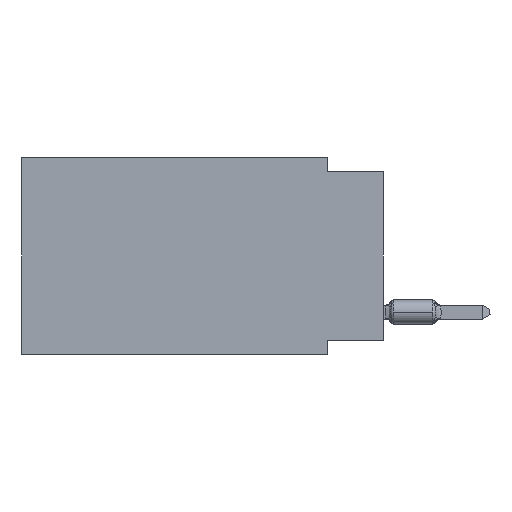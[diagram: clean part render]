
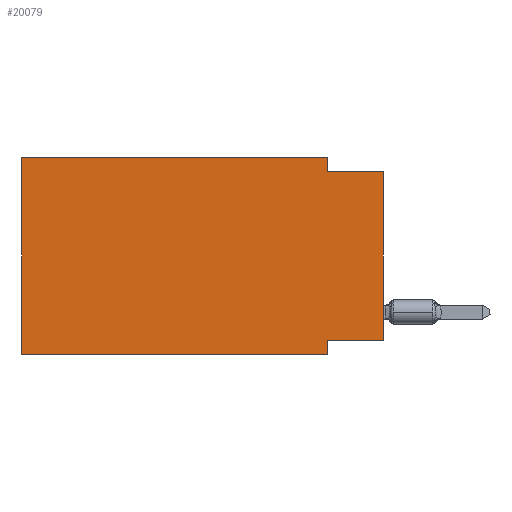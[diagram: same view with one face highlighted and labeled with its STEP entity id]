
A CAD part, left-side view. The second image highlights one B-rep face of the part: STEP entity #20079.
In plain terms, the highlighted planar face has unit normal (-1, 0, 0).
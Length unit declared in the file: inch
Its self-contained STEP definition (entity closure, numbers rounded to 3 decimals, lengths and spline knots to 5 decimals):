
#192 = DIRECTION ( 'NONE',  ( 0., 0., 1. ) ) ;
#634 = DIRECTION ( 'NONE',  ( 1., 0., 0. ) ) ;
#734 = ORIENTED_EDGE ( 'NONE', *, *, #3717, .T. ) ;
#810 = DIRECTION ( 'NONE',  ( 0., -1., 0. ) ) ;
#1133 = CARTESIAN_POINT ( 'NONE',  ( 0., 0.1, -0.35 ) ) ;
#1271 = ORIENTED_EDGE ( 'NONE', *, *, #18284, .F. ) ;
#1396 = DIRECTION ( 'NONE',  ( 0., 0., -1. ) ) ;
#1654 = VECTOR ( 'NONE', #6037, 39.37008 ) ;
#2083 = CARTESIAN_POINT ( 'NONE',  ( 0., 0.1, 0. ) ) ;
#3013 = LINE ( 'NONE', #26594, #38229 ) ;
#3106 = DIRECTION ( 'NONE',  ( 0., 1., 0. ) ) ;
#3715 = CARTESIAN_POINT ( 'NONE',  ( 0., 0.645, 0. ) ) ;
#3717 = EDGE_CURVE ( 'NONE', #37542, #27082, #29189, .T. ) ;
#5057 = LINE ( 'NONE', #32668, #30152 ) ;
#5499 = VECTOR ( 'NONE', #810, 39.37008 ) ;
#6037 = DIRECTION ( 'NONE',  ( 0., 0., -1. ) ) ;
#6603 = PLANE ( 'NONE',  #20272 ) ;
#6747 = ORIENTED_EDGE ( 'NONE', *, *, #32597, .F. ) ;
#7682 = ORIENTED_EDGE ( 'NONE', *, *, #27638, .F. ) ;
#8746 = CARTESIAN_POINT ( 'NONE',  ( 0., 0., -0.325 ) ) ;
#9188 = LINE ( 'NONE', #30029, #36818 ) ;
#9870 = CARTESIAN_POINT ( 'NONE',  ( 0., 0.1, -0.025 ) ) ;
#10461 = VECTOR ( 'NONE', #13053, 39.37008 ) ;
#11856 = EDGE_LOOP ( 'NONE', ( #734, #6747, #25979, #7682, #1271, #34753, #24120, #24222 ) ) ;
#12015 = VERTEX_POINT ( 'NONE', #1133 ) ;
#13053 = DIRECTION ( 'NONE',  ( 0., 0., -1. ) ) ;
#13111 = CARTESIAN_POINT ( 'NONE',  ( 0., 0.1, -0.325 ) ) ;
#14891 = CARTESIAN_POINT ( 'NONE',  ( 0., 0., 0. ) ) ;
#14967 = VERTEX_POINT ( 'NONE', #9870 ) ;
#15147 = LINE ( 'NONE', #32734, #25679 ) ;
#15160 = DIRECTION ( 'NONE',  ( 0., 0., 1. ) ) ;
#15485 = VERTEX_POINT ( 'NONE', #13111 ) ;
#18284 = EDGE_CURVE ( 'NONE', #34834, #24969, #9188, .T. ) ;
#18789 = FACE_OUTER_BOUND ( 'NONE', #11856, .T. ) ;
#19514 = CARTESIAN_POINT ( 'NONE',  ( 0., 0., -0.025 ) ) ;
#20079 = ADVANCED_FACE ( 'NONE', ( #18789 ), #6603, .F. ) ;
#20272 = AXIS2_PLACEMENT_3D ( 'NONE', #3715, #634, #1396 ) ;
#20387 = EDGE_CURVE ( 'NONE', #37542, #15485, #5057, .T. ) ;
#21879 = VECTOR ( 'NONE', #192, 39.37008 ) ;
#23506 = DIRECTION ( 'NONE',  ( 0., -1., 0. ) ) ;
#24120 = ORIENTED_EDGE ( 'NONE', *, *, #32809, .F. ) ;
#24222 = ORIENTED_EDGE ( 'NONE', *, *, #20387, .F. ) ;
#24710 = EDGE_CURVE ( 'NONE', #36396, #14967, #29805, .T. ) ;
#24969 = VERTEX_POINT ( 'NONE', #29521 ) ;
#25596 = CARTESIAN_POINT ( 'NONE',  ( 0., 0.1, -0.35 ) ) ;
#25679 = VECTOR ( 'NONE', #36397, 39.37008 ) ;
#25979 = ORIENTED_EDGE ( 'NONE', *, *, #24710, .F. ) ;
#26594 = CARTESIAN_POINT ( 'NONE',  ( 0., 0., -0.025 ) ) ;
#27082 = VERTEX_POINT ( 'NONE', #19514 ) ;
#27638 = EDGE_CURVE ( 'NONE', #24969, #36396, #15147, .T. ) ;
#28114 = LINE ( 'NONE', #25596, #10461 ) ;
#28678 = CARTESIAN_POINT ( 'NONE',  ( 0., 0.645, -0.35 ) ) ;
#29189 = LINE ( 'NONE', #14891, #21879 ) ;
#29426 = CARTESIAN_POINT ( 'NONE',  ( 0., 0.1, 0. ) ) ;
#29521 = CARTESIAN_POINT ( 'NONE',  ( 0., 0.645, 0. ) ) ;
#29805 = LINE ( 'NONE', #29426, #1654 ) ;
#30029 = CARTESIAN_POINT ( 'NONE',  ( 0., 0.645, 0. ) ) ;
#30152 = VECTOR ( 'NONE', #3106, 39.37008 ) ;
#30561 = CARTESIAN_POINT ( 'NONE',  ( 0., 0.645, -0.35 ) ) ;
#30782 = EDGE_CURVE ( 'NONE', #34834, #12015, #33280, .T. ) ;
#32597 = EDGE_CURVE ( 'NONE', #14967, #27082, #3013, .T. ) ;
#32668 = CARTESIAN_POINT ( 'NONE',  ( 0., 0., -0.325 ) ) ;
#32734 = CARTESIAN_POINT ( 'NONE',  ( 0., 0.645, 0. ) ) ;
#32809 = EDGE_CURVE ( 'NONE', #15485, #12015, #28114, .T. ) ;
#33280 = LINE ( 'NONE', #30561, #5499 ) ;
#34753 = ORIENTED_EDGE ( 'NONE', *, *, #30782, .T. ) ;
#34834 = VERTEX_POINT ( 'NONE', #28678 ) ;
#36396 = VERTEX_POINT ( 'NONE', #2083 ) ;
#36397 = DIRECTION ( 'NONE',  ( 0., -1., 0. ) ) ;
#36818 = VECTOR ( 'NONE', #15160, 39.37008 ) ;
#37542 = VERTEX_POINT ( 'NONE', #8746 ) ;
#38229 = VECTOR ( 'NONE', #23506, 39.37008 ) ;
